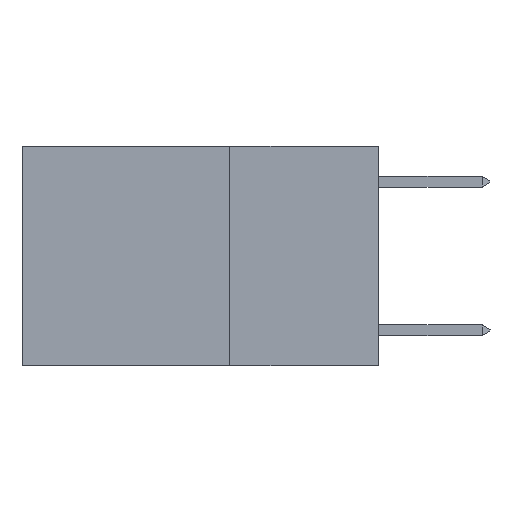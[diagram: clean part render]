
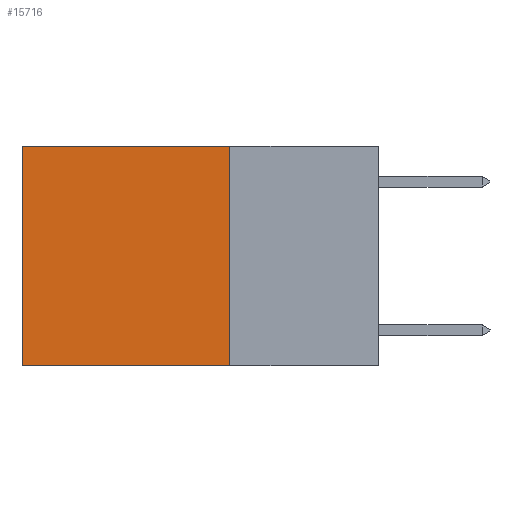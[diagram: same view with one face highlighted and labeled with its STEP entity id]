
A CAD part, left-side view. The second image highlights one B-rep face of the part: STEP entity #15716.
In plain terms, the highlighted planar face has unit normal (-1, 0, 0).
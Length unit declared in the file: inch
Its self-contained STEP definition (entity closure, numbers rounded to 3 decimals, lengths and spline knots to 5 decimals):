
#143 = PLANE ( 'NONE',  #9772 ) ;
#999 = VERTEX_POINT ( 'NONE', #26455 ) ;
#1440 = ORIENTED_EDGE ( 'NONE', *, *, #5616, .T. ) ;
#2000 = CARTESIAN_POINT ( 'NONE',  ( 0.2625, 0.6, -0.37 ) ) ;
#2354 = CARTESIAN_POINT ( 'NONE',  ( 0.2625, 0.6, 0. ) ) ;
#2373 = DIRECTION ( 'NONE',  ( 1., 0., 0. ) ) ;
#4233 = VERTEX_POINT ( 'NONE', #25436 ) ;
#4540 = EDGE_CURVE ( 'NONE', #999, #4233, #7838, .T. ) ;
#4575 = DIRECTION ( 'NONE',  ( 0., 0., -1. ) ) ;
#5051 = CARTESIAN_POINT ( 'NONE',  ( 0.2625, 0.25, -0.37 ) ) ;
#5474 = ORIENTED_EDGE ( 'NONE', *, *, #12936, .F. ) ;
#5616 = EDGE_CURVE ( 'NONE', #999, #7149, #24768, .T. ) ;
#7149 = VERTEX_POINT ( 'NONE', #7926 ) ;
#7239 = DIRECTION ( 'NONE',  ( 0., 1., 0. ) ) ;
#7511 = VECTOR ( 'NONE', #4575, 39.37008 ) ;
#7782 = VECTOR ( 'NONE', #18295, 39.37008 ) ;
#7838 = LINE ( 'NONE', #16317, #7782 ) ;
#7926 = CARTESIAN_POINT ( 'NONE',  ( 0.2625, 0.6, 0. ) ) ;
#8771 = ORIENTED_EDGE ( 'NONE', *, *, #19862, .T. ) ;
#9772 = AXIS2_PLACEMENT_3D ( 'NONE', #14874, #2373, #16914 ) ;
#12634 = VERTEX_POINT ( 'NONE', #2000 ) ;
#12936 = EDGE_CURVE ( 'NONE', #4233, #12634, #22489, .T. ) ;
#13313 = CARTESIAN_POINT ( 'NONE',  ( 0.2625, 0.25, 0. ) ) ;
#14704 = FACE_OUTER_BOUND ( 'NONE', #22779, .T. ) ;
#14874 = CARTESIAN_POINT ( 'NONE',  ( 0.2625, 0.25, 0. ) ) ;
#15716 = ADVANCED_FACE ( 'NONE', ( #14704 ), #143, .F. ) ;
#16317 = CARTESIAN_POINT ( 'NONE',  ( 0.2625, 0.25, 0. ) ) ;
#16914 = DIRECTION ( 'NONE',  ( 0., 0., -1. ) ) ;
#18295 = DIRECTION ( 'NONE',  ( 0., 0., -1. ) ) ;
#19862 = EDGE_CURVE ( 'NONE', #7149, #12634, #20152, .T. ) ;
#20152 = LINE ( 'NONE', #2354, #7511 ) ;
#22380 = VECTOR ( 'NONE', #7239, 39.37008 ) ;
#22489 = LINE ( 'NONE', #5051, #22380 ) ;
#22779 = EDGE_LOOP ( 'NONE', ( #8771, #5474, #23134, #1440 ) ) ;
#23134 = ORIENTED_EDGE ( 'NONE', *, *, #4540, .F. ) ;
#24768 = LINE ( 'NONE', #13313, #25023 ) ;
#25023 = VECTOR ( 'NONE', #25380, 39.37008 ) ;
#25380 = DIRECTION ( 'NONE',  ( 0., 1., 0. ) ) ;
#25436 = CARTESIAN_POINT ( 'NONE',  ( 0.2625, 0.25, -0.37 ) ) ;
#26455 = CARTESIAN_POINT ( 'NONE',  ( 0.2625, 0.25, 0. ) ) ;
